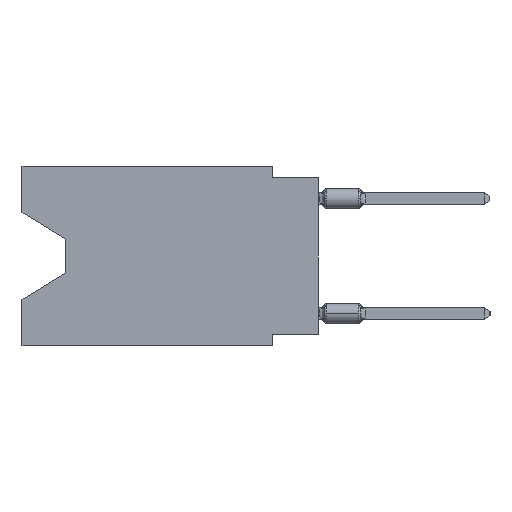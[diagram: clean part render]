
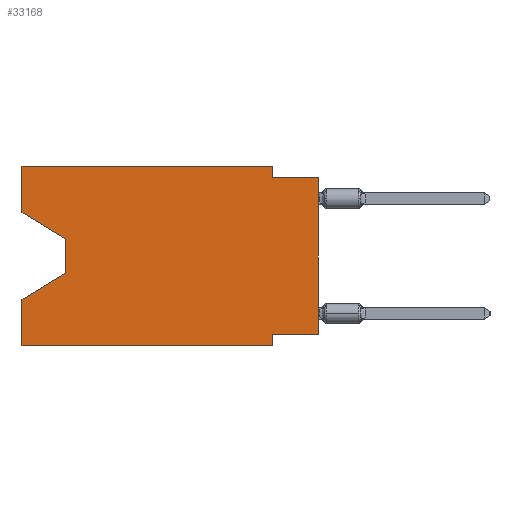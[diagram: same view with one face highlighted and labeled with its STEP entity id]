
A CAD part, left-side view. The second image highlights one B-rep face of the part: STEP entity #33168.
In plain terms, the highlighted planar face has unit normal (-1, 0, 0).
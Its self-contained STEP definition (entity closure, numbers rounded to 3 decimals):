
#711 = AXIS2_PLACEMENT_3D ( 'NONE', #793, #9633, #2481 ) ;
#793 = CARTESIAN_POINT ( 'NONE',  ( 0., 16.383, 0. ) ) ;
#1698 = VECTOR ( 'NONE', #41064, 1000. ) ;
#2481 = DIRECTION ( 'NONE',  ( 0., 0., -1. ) ) ;
#3470 = ORIENTED_EDGE ( 'NONE', *, *, #12835, .F. ) ;
#6266 = VECTOR ( 'NONE', #14088, 1000. ) ;
#6300 = EDGE_CURVE ( 'NONE', #32792, #53227, #16145, .T. ) ;
#6467 = LINE ( 'NONE', #24427, #24845 ) ;
#7217 = VERTEX_POINT ( 'NONE', #22528 ) ;
#7367 = ORIENTED_EDGE ( 'NONE', *, *, #21567, .T. ) ;
#7498 = LINE ( 'NONE', #12604, #33459 ) ;
#8143 = CARTESIAN_POINT ( 'NONE',  ( 0., 16.383, -9.906 ) ) ;
#9633 = DIRECTION ( 'NONE',  ( 1., 0., 0. ) ) ;
#9718 = VERTEX_POINT ( 'NONE', #8143 ) ;
#10512 = ORIENTED_EDGE ( 'NONE', *, *, #43470, .F. ) ;
#10532 = CARTESIAN_POINT ( 'NONE',  ( 0., 0., -0.635 ) ) ;
#10933 = LINE ( 'NONE', #36087, #37313 ) ;
#11104 = ORIENTED_EDGE ( 'NONE', *, *, #52972, .T. ) ;
#11407 = CARTESIAN_POINT ( 'NONE',  ( 0., 2.54, -0.635 ) ) ;
#11438 = LINE ( 'NONE', #38008, #37871 ) ;
#11622 = CARTESIAN_POINT ( 'NONE',  ( 0., 13.97, -4.013 ) ) ;
#12025 = LINE ( 'NONE', #46883, #55719 ) ;
#12604 = CARTESIAN_POINT ( 'NONE',  ( 0., 2.54, -9.906 ) ) ;
#12835 = EDGE_CURVE ( 'NONE', #18200, #54803, #11438, .T. ) ;
#13276 = CARTESIAN_POINT ( 'NONE',  ( 0., 16.383, 0. ) ) ;
#13781 = DIRECTION ( 'NONE',  ( 0., -1., 0. ) ) ;
#14088 = DIRECTION ( 'NONE',  ( 0., 0.855, -0.519 ) ) ;
#14835 = DIRECTION ( 'NONE',  ( 0., -1., 0. ) ) ;
#15860 = VECTOR ( 'NONE', #14835, 1000. ) ;
#16055 = DIRECTION ( 'NONE',  ( 0., 0., -1. ) ) ;
#16145 = LINE ( 'NONE', #56104, #37336 ) ;
#17529 = CARTESIAN_POINT ( 'NONE',  ( 0., 13.97, -5.893 ) ) ;
#18200 = VERTEX_POINT ( 'NONE', #54483 ) ;
#18615 = CARTESIAN_POINT ( 'NONE',  ( 0., 16.383, -9.906 ) ) ;
#18686 = ORIENTED_EDGE ( 'NONE', *, *, #6300, .T. ) ;
#18987 = LINE ( 'NONE', #23838, #37089 ) ;
#21567 = EDGE_CURVE ( 'NONE', #53227, #56132, #39240, .T. ) ;
#22528 = CARTESIAN_POINT ( 'NONE',  ( 0., 2.54, -9.906 ) ) ;
#23278 = DIRECTION ( 'NONE',  ( 0., 0., 1. ) ) ;
#23580 = DIRECTION ( 'NONE',  ( 0., 0., -1. ) ) ;
#23838 = CARTESIAN_POINT ( 'NONE',  ( 0., 16.383, 0. ) ) ;
#24427 = CARTESIAN_POINT ( 'NONE',  ( 0., 2.54, 0. ) ) ;
#24494 = CARTESIAN_POINT ( 'NONE',  ( 0., 0., -9.271 ) ) ;
#24585 = DIRECTION ( 'NONE',  ( 0., 0., 1. ) ) ;
#24845 = VECTOR ( 'NONE', #23580, 1000. ) ;
#25161 = DIRECTION ( 'NONE',  ( 0., -1., 0. ) ) ;
#26420 = ORIENTED_EDGE ( 'NONE', *, *, #47829, .T. ) ;
#29619 = LINE ( 'NONE', #37922, #43031 ) ;
#30079 = VERTEX_POINT ( 'NONE', #53834 ) ;
#30746 = CARTESIAN_POINT ( 'NONE',  ( 0., 13.97, -5.893 ) ) ;
#31422 = EDGE_CURVE ( 'NONE', #9718, #56132, #18987, .T. ) ;
#31999 = EDGE_CURVE ( 'NONE', #53352, #7217, #7498, .T. ) ;
#32076 = CARTESIAN_POINT ( 'NONE',  ( 0., 0., -0.635 ) ) ;
#32162 = CARTESIAN_POINT ( 'NONE',  ( 0., 2.54, -9.271 ) ) ;
#32756 = ORIENTED_EDGE ( 'NONE', *, *, #53288, .F. ) ;
#32792 = VERTEX_POINT ( 'NONE', #11622 ) ;
#32793 = LINE ( 'NONE', #24494, #1698 ) ;
#33168 = ADVANCED_FACE ( 'NONE', ( #39907 ), #53046, .F. ) ;
#33459 = VECTOR ( 'NONE', #16055, 1000. ) ;
#34434 = CARTESIAN_POINT ( 'NONE',  ( 0., 0., -9.271 ) ) ;
#35709 = VERTEX_POINT ( 'NONE', #11407 ) ;
#35791 = ORIENTED_EDGE ( 'NONE', *, *, #49169, .T. ) ;
#36087 = CARTESIAN_POINT ( 'NONE',  ( 0., 16.383, -2.546 ) ) ;
#36792 = ORIENTED_EDGE ( 'NONE', *, *, #31999, .F. ) ;
#36861 = ORIENTED_EDGE ( 'NONE', *, *, #46657, .F. ) ;
#36946 = VECTOR ( 'NONE', #13781, 1000. ) ;
#36962 = CARTESIAN_POINT ( 'NONE',  ( 0., 16.383, -7.36 ) ) ;
#37089 = VECTOR ( 'NONE', #23278, 1000. ) ;
#37313 = VECTOR ( 'NONE', #53503, 1000. ) ;
#37336 = VECTOR ( 'NONE', #51833, 1000. ) ;
#37871 = VECTOR ( 'NONE', #24585, 1000. ) ;
#37922 = CARTESIAN_POINT ( 'NONE',  ( 0., 0., 0. ) ) ;
#38008 = CARTESIAN_POINT ( 'NONE',  ( 0., 16.383, 0. ) ) ;
#39240 = LINE ( 'NONE', #17529, #6266 ) ;
#39907 = FACE_OUTER_BOUND ( 'NONE', #42458, .T. ) ;
#40175 = EDGE_CURVE ( 'NONE', #41662, #53352, #32793, .T. ) ;
#41064 = DIRECTION ( 'NONE',  ( 0., 1., 0. ) ) ;
#41662 = VERTEX_POINT ( 'NONE', #34434 ) ;
#42458 = EDGE_LOOP ( 'NONE', ( #35791, #18686, #7367, #53468, #26420, #36792, #43853, #11104, #36861, #32756, #10512, #3470 ) ) ;
#43031 = VECTOR ( 'NONE', #47334, 1000. ) ;
#43470 = EDGE_CURVE ( 'NONE', #54803, #30079, #12025, .T. ) ;
#43853 = ORIENTED_EDGE ( 'NONE', *, *, #40175, .F. ) ;
#46657 = EDGE_CURVE ( 'NONE', #35709, #49053, #49385, .T. ) ;
#46883 = CARTESIAN_POINT ( 'NONE',  ( 0., 16.383, 0. ) ) ;
#47334 = DIRECTION ( 'NONE',  ( 0., 0., 1. ) ) ;
#47829 = EDGE_CURVE ( 'NONE', #9718, #7217, #52617, .T. ) ;
#49053 = VERTEX_POINT ( 'NONE', #32076 ) ;
#49169 = EDGE_CURVE ( 'NONE', #18200, #32792, #10933, .T. ) ;
#49385 = LINE ( 'NONE', #10532, #15860 ) ;
#51833 = DIRECTION ( 'NONE',  ( 0., 0., -1. ) ) ;
#52617 = LINE ( 'NONE', #18615, #36946 ) ;
#52972 = EDGE_CURVE ( 'NONE', #41662, #49053, #29619, .T. ) ;
#53046 = PLANE ( 'NONE',  #711 ) ;
#53227 = VERTEX_POINT ( 'NONE', #30746 ) ;
#53288 = EDGE_CURVE ( 'NONE', #30079, #35709, #6467, .T. ) ;
#53352 = VERTEX_POINT ( 'NONE', #32162 ) ;
#53468 = ORIENTED_EDGE ( 'NONE', *, *, #31422, .F. ) ;
#53503 = DIRECTION ( 'NONE',  ( 0., -0.855, -0.519 ) ) ;
#53834 = CARTESIAN_POINT ( 'NONE',  ( 0., 2.54, 0. ) ) ;
#54483 = CARTESIAN_POINT ( 'NONE',  ( 0., 16.383, -2.546 ) ) ;
#54803 = VERTEX_POINT ( 'NONE', #13276 ) ;
#55719 = VECTOR ( 'NONE', #25161, 1000. ) ;
#56104 = CARTESIAN_POINT ( 'NONE',  ( 0., 13.97, -4.013 ) ) ;
#56132 = VERTEX_POINT ( 'NONE', #36962 ) ;
